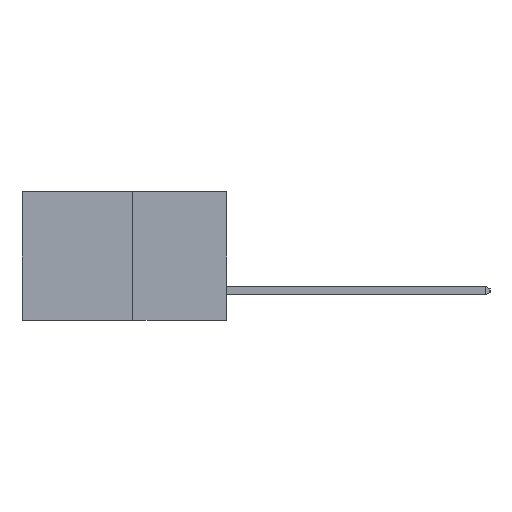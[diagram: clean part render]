
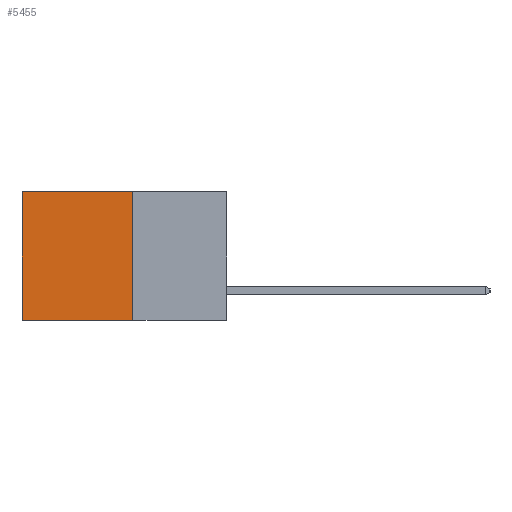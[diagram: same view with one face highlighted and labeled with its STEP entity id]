
A CAD part, left-side view. The second image highlights one B-rep face of the part: STEP entity #5455.
In plain terms, the highlighted planar face has unit normal (-1, 0, 0).
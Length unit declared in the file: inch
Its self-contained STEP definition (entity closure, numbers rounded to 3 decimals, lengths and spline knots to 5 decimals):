
#147 = DIRECTION ( 'NONE',  ( 0., 1., 0. ) ) ;
#712 = VERTEX_POINT ( 'NONE', #9721 ) ;
#904 = ORIENTED_EDGE ( 'NONE', *, *, #10288, .F. ) ;
#947 = VECTOR ( 'NONE', #6410, 39.37008 ) ;
#1762 = CARTESIAN_POINT ( 'NONE',  ( 0.277, 0.27, 0. ) ) ;
#1970 = ORIENTED_EDGE ( 'NONE', *, *, #9476, .F. ) ;
#3582 = EDGE_CURVE ( 'NONE', #6571, #5356, #10683, .T. ) ;
#3892 = ORIENTED_EDGE ( 'NONE', *, *, #3582, .T. ) ;
#4333 = EDGE_LOOP ( 'NONE', ( #6164, #1970, #904, #3892 ) ) ;
#5356 = VERTEX_POINT ( 'NONE', #7078 ) ;
#5357 = DIRECTION ( 'NONE',  ( 0., 0., -1. ) ) ;
#5455 = ADVANCED_FACE ( 'NONE', ( #9945 ), #5854, .F. ) ;
#5794 = DIRECTION ( 'NONE',  ( 0., 0., -1. ) ) ;
#5797 = DIRECTION ( 'NONE',  ( 1., 0., 0. ) ) ;
#5854 = PLANE ( 'NONE',  #8991 ) ;
#5870 = CARTESIAN_POINT ( 'NONE',  ( 0.277, 0.27, -0.37 ) ) ;
#5925 = CARTESIAN_POINT ( 'NONE',  ( 0.277, 0.27, 0. ) ) ;
#6164 = ORIENTED_EDGE ( 'NONE', *, *, #7268, .T. ) ;
#6196 = CARTESIAN_POINT ( 'NONE',  ( 0.277, 0.27, -0.37 ) ) ;
#6410 = DIRECTION ( 'NONE',  ( 0., 1., 0. ) ) ;
#6571 = VERTEX_POINT ( 'NONE', #5925 ) ;
#6582 = LINE ( 'NONE', #10863, #10532 ) ;
#7003 = DIRECTION ( 'NONE',  ( 0., 0., -1. ) ) ;
#7078 = CARTESIAN_POINT ( 'NONE',  ( 0.277, 0.59, 0. ) ) ;
#7199 = VERTEX_POINT ( 'NONE', #8629 ) ;
#7268 = EDGE_CURVE ( 'NONE', #5356, #7199, #8594, .T. ) ;
#8594 = LINE ( 'NONE', #10478, #11116 ) ;
#8629 = CARTESIAN_POINT ( 'NONE',  ( 0.277, 0.59, -0.37 ) ) ;
#8991 = AXIS2_PLACEMENT_3D ( 'NONE', #5870, #5797, #5794 ) ;
#9416 = VECTOR ( 'NONE', #7003, 39.37008 ) ;
#9476 = EDGE_CURVE ( 'NONE', #712, #7199, #6582, .T. ) ;
#9671 = LINE ( 'NONE', #6196, #9416 ) ;
#9721 = CARTESIAN_POINT ( 'NONE',  ( 0.277, 0.27, -0.37 ) ) ;
#9945 = FACE_OUTER_BOUND ( 'NONE', #4333, .T. ) ;
#10288 = EDGE_CURVE ( 'NONE', #6571, #712, #9671, .T. ) ;
#10478 = CARTESIAN_POINT ( 'NONE',  ( 0.277, 0.59, -0.37 ) ) ;
#10532 = VECTOR ( 'NONE', #147, 39.37008 ) ;
#10683 = LINE ( 'NONE', #1762, #947 ) ;
#10863 = CARTESIAN_POINT ( 'NONE',  ( 0.277, 0.27, -0.37 ) ) ;
#11116 = VECTOR ( 'NONE', #5357, 39.37008 ) ;
